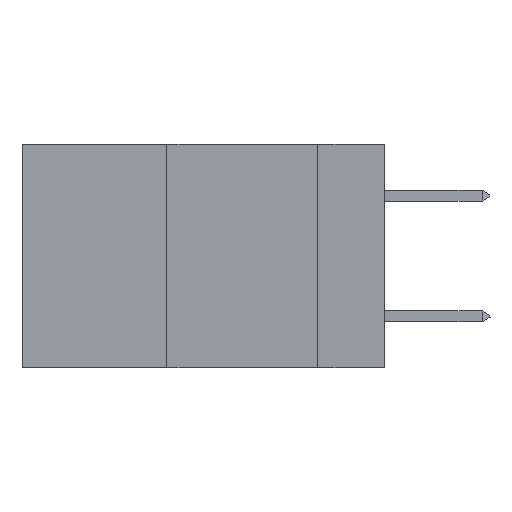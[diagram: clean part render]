
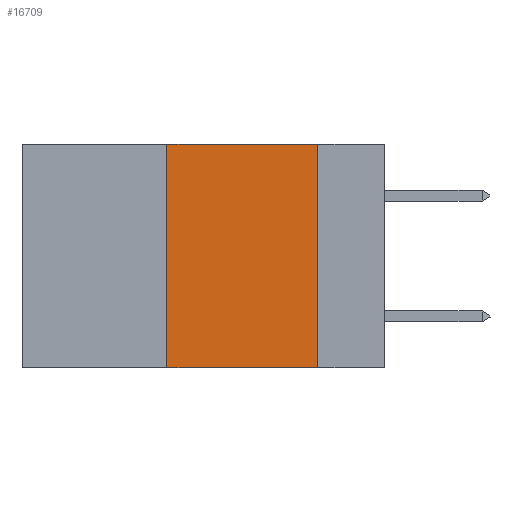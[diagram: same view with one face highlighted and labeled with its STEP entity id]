
A CAD part, left-side view. The second image highlights one B-rep face of the part: STEP entity #16709.
In plain terms, the highlighted planar face has unit normal (-1, 0, 0).
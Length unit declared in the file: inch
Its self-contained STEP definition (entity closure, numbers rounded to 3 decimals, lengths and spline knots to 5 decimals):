
#351 = CARTESIAN_POINT ( 'NONE',  ( 0., 0.11, 0. ) ) ;
#432 = EDGE_CURVE ( 'NONE', #11436, #19225, #19400, .T. ) ;
#862 = CARTESIAN_POINT ( 'NONE',  ( 0., 0.36, -0.37 ) ) ;
#1182 = ORIENTED_EDGE ( 'NONE', *, *, #432, .F. ) ;
#1798 = EDGE_LOOP ( 'NONE', ( #6546, #1182, #10980, #13687 ) ) ;
#1895 = CARTESIAN_POINT ( 'NONE',  ( 0., 0.6, 0. ) ) ;
#3530 = DIRECTION ( 'NONE',  ( 1., 0., 0. ) ) ;
#3536 = CARTESIAN_POINT ( 'NONE',  ( 0., 0.36, 0. ) ) ;
#3613 = VECTOR ( 'NONE', #5064, 39.37008 ) ;
#4361 = EDGE_CURVE ( 'NONE', #4430, #11070, #17811, .T. ) ;
#4430 = VERTEX_POINT ( 'NONE', #862 ) ;
#5064 = DIRECTION ( 'NONE',  ( 0., 0., -1. ) ) ;
#6546 = ORIENTED_EDGE ( 'NONE', *, *, #14302, .F. ) ;
#8214 = AXIS2_PLACEMENT_3D ( 'NONE', #1895, #3530, #14321 ) ;
#8238 = LINE ( 'NONE', #14769, #15738 ) ;
#10253 = EDGE_CURVE ( 'NONE', #4430, #11436, #8238, .T. ) ;
#10526 = CARTESIAN_POINT ( 'NONE',  ( 0., 0.11, -0.37 ) ) ;
#10980 = ORIENTED_EDGE ( 'NONE', *, *, #10253, .F. ) ;
#11070 = VERTEX_POINT ( 'NONE', #10526 ) ;
#11436 = VERTEX_POINT ( 'NONE', #3536 ) ;
#12852 = PLANE ( 'NONE',  #8214 ) ;
#13396 = CARTESIAN_POINT ( 'NONE',  ( 0., 0.6, 0. ) ) ;
#13687 = ORIENTED_EDGE ( 'NONE', *, *, #4361, .T. ) ;
#14107 = VECTOR ( 'NONE', #15694, 39.37008 ) ;
#14302 = EDGE_CURVE ( 'NONE', #19225, #11070, #18972, .T. ) ;
#14321 = DIRECTION ( 'NONE',  ( 0., 0., -1. ) ) ;
#14769 = CARTESIAN_POINT ( 'NONE',  ( 0., 0.36, 0. ) ) ;
#15348 = VECTOR ( 'NONE', #16505, 39.37008 ) ;
#15694 = DIRECTION ( 'NONE',  ( 0., -1., 0. ) ) ;
#15738 = VECTOR ( 'NONE', #18857, 39.37008 ) ;
#16505 = DIRECTION ( 'NONE',  ( 0., -1., 0. ) ) ;
#16709 = ADVANCED_FACE ( 'NONE', ( #17644 ), #12852, .F. ) ;
#16995 = CARTESIAN_POINT ( 'NONE',  ( 0., 0.6, -0.37 ) ) ;
#17644 = FACE_OUTER_BOUND ( 'NONE', #1798, .T. ) ;
#17811 = LINE ( 'NONE', #16995, #14107 ) ;
#18465 = CARTESIAN_POINT ( 'NONE',  ( 0., 0.11, 0. ) ) ;
#18857 = DIRECTION ( 'NONE',  ( 0., 0., 1. ) ) ;
#18972 = LINE ( 'NONE', #18465, #3613 ) ;
#19225 = VERTEX_POINT ( 'NONE', #351 ) ;
#19400 = LINE ( 'NONE', #13396, #15348 ) ;
